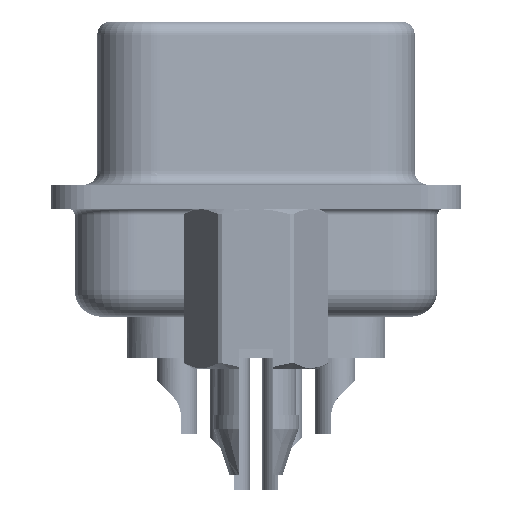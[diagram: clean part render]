
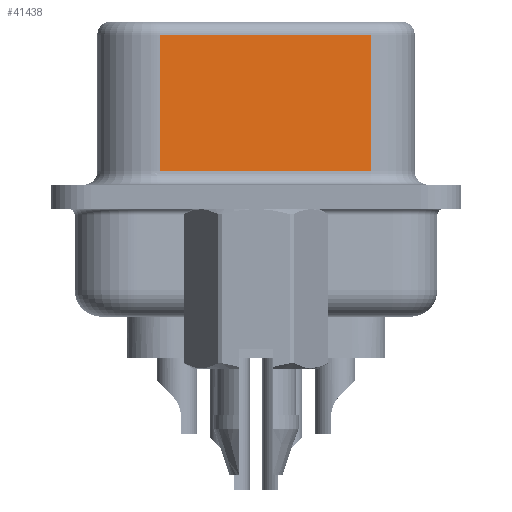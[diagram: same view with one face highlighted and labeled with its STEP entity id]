
A CAD part, left-side view. The second image highlights one B-rep face of the part: STEP entity #41438.
In plain terms, the highlighted planar face has unit normal (-0.985, -0.174, 0).
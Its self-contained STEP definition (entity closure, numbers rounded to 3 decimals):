
#2655 = DIRECTION ( 'NONE',  ( 0.985, 0.174, 0. ) ) ;
#3048 = EDGE_CURVE ( 'NONE', #38347, #18215, #42122, .T. ) ;
#3511 = CARTESIAN_POINT ( 'NONE',  ( 5.128, -4.297, 6.57 ) ) ;
#6594 = VECTOR ( 'NONE', #38907, 1000. ) ;
#9339 = EDGE_CURVE ( 'NONE', #36015, #38347, #19299, .T. ) ;
#10877 = AXIS2_PLACEMENT_3D ( 'NONE', #3511, #2655, #12528 ) ;
#12484 = VECTOR ( 'NONE', #39083, 1000. ) ;
#12528 = DIRECTION ( 'NONE',  ( -0.174, 0.985, 0. ) ) ;
#13028 = DIRECTION ( 'NONE',  ( 0., 0., -1. ) ) ;
#13059 = CARTESIAN_POINT ( 'NONE',  ( 5.128, -4.297, 0.95 ) ) ;
#15415 = CARTESIAN_POINT ( 'NONE',  ( 3.735, 3.603, 6.07 ) ) ;
#18215 = VERTEX_POINT ( 'NONE', #13059 ) ;
#19299 = LINE ( 'NONE', #19505, #29524 ) ;
#19505 = CARTESIAN_POINT ( 'NONE',  ( 3.735, 3.603, 6.57 ) ) ;
#20045 = CARTESIAN_POINT ( 'NONE',  ( 3.735, 3.603, 0.95 ) ) ;
#20391 = ORIENTED_EDGE ( 'NONE', *, *, #22983, .T. ) ;
#21448 = LINE ( 'NONE', #35480, #22924 ) ;
#22014 = CARTESIAN_POINT ( 'NONE',  ( 5.128, -4.297, 6.07 ) ) ;
#22924 = VECTOR ( 'NONE', #41996, 1000. ) ;
#22983 = EDGE_CURVE ( 'NONE', #33875, #36015, #21448, .T. ) ;
#23425 = ORIENTED_EDGE ( 'NONE', *, *, #27613, .F. ) ;
#25709 = CARTESIAN_POINT ( 'NONE',  ( 5.128, -4.297, 6.57 ) ) ;
#26425 = PLANE ( 'NONE',  #10877 ) ;
#27342 = EDGE_LOOP ( 'NONE', ( #23425, #20391, #31678, #36293 ) ) ;
#27613 = EDGE_CURVE ( 'NONE', #33875, #18215, #39125, .T. ) ;
#29524 = VECTOR ( 'NONE', #13028, 1000. ) ;
#31678 = ORIENTED_EDGE ( 'NONE', *, *, #9339, .T. ) ;
#33875 = VERTEX_POINT ( 'NONE', #22014 ) ;
#34548 = CARTESIAN_POINT ( 'NONE',  ( 5.128, -4.297, 0.95 ) ) ;
#35480 = CARTESIAN_POINT ( 'NONE',  ( 5.128, -4.297, 6.07 ) ) ;
#36015 = VERTEX_POINT ( 'NONE', #15415 ) ;
#36156 = FACE_OUTER_BOUND ( 'NONE', #27342, .T. ) ;
#36293 = ORIENTED_EDGE ( 'NONE', *, *, #3048, .T. ) ;
#38347 = VERTEX_POINT ( 'NONE', #20045 ) ;
#38907 = DIRECTION ( 'NONE',  ( 0., 0., -1. ) ) ;
#39083 = DIRECTION ( 'NONE',  ( 0.174, -0.985, 0. ) ) ;
#39125 = LINE ( 'NONE', #25709, #6594 ) ;
#41438 = ADVANCED_FACE ( 'NONE', ( #36156 ), #26425, .F. ) ;
#41996 = DIRECTION ( 'NONE',  ( -0.174, 0.985, 0. ) ) ;
#42122 = LINE ( 'NONE', #34548, #12484 ) ;
